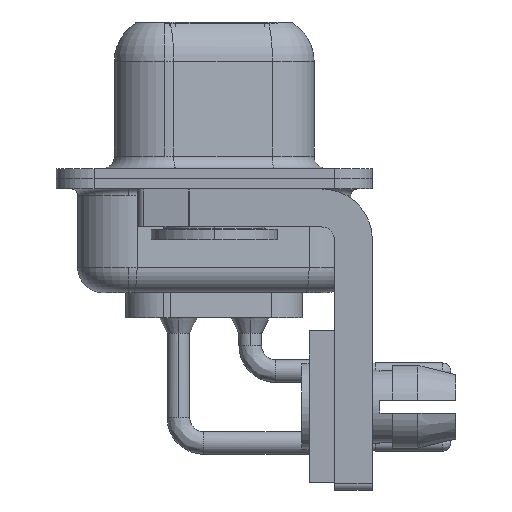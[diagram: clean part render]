
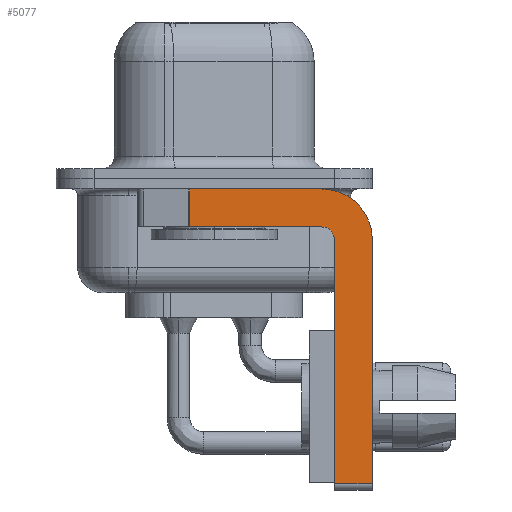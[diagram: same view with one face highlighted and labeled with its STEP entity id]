
A CAD part, left-side view. The second image highlights one B-rep face of the part: STEP entity #5077.
In plain terms, the highlighted planar face has unit normal (-1, 0, 0).
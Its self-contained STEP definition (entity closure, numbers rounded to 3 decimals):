
#413 = DIRECTION ( 'NONE',  ( 0., -1., 0. ) ) ;
#438 = EDGE_CURVE ( 'NONE', #1953, #17563, #21297, .T. ) ;
#476 = AXIS2_PLACEMENT_3D ( 'NONE', #9005, #9037, #8812 ) ;
#985 = CIRCLE ( 'NONE', #476, 2. ) ;
#1953 = VERTEX_POINT ( 'NONE', #21145 ) ;
#1963 = EDGE_CURVE ( 'NONE', #9239, #7522, #6109, .T. ) ;
#2119 = AXIS2_PLACEMENT_3D ( 'NONE', #20355, #21916, #20970 ) ;
#2175 = EDGE_CURVE ( 'NONE', #17563, #11756, #985, .T. ) ;
#2285 = LINE ( 'NONE', #16053, #13680 ) ;
#2563 = DIRECTION ( 'NONE',  ( 0., 0., -1. ) ) ;
#2625 = CARTESIAN_POINT ( 'NONE',  ( -2.9, -4.25, -0.4 ) ) ;
#2735 = VERTEX_POINT ( 'NONE', #4175 ) ;
#3750 = VECTOR ( 'NONE', #413, 1000. ) ;
#3784 = ORIENTED_EDGE ( 'NONE', *, *, #438, .F. ) ;
#3963 = EDGE_CURVE ( 'NONE', #6126, #12973, #21067, .T. ) ;
#4175 = CARTESIAN_POINT ( 'NONE',  ( -2.9, 0.978, -1.9 ) ) ;
#5077 = ADVANCED_FACE ( 'NONE', ( #16055 ), #5805, .F. ) ;
#5805 = PLANE ( 'NONE',  #9897 ) ;
#5872 = CARTESIAN_POINT ( 'NONE',  ( -2.9, -4.25, -2.4 ) ) ;
#6109 = CIRCLE ( 'NONE', #2119, 0.5 ) ;
#6126 = VERTEX_POINT ( 'NONE', #13852 ) ;
#6185 = DIRECTION ( 'NONE',  ( 0., 0., -1. ) ) ;
#6246 = DIRECTION ( 'NONE',  ( 1., 0., 0. ) ) ;
#6456 = ORIENTED_EDGE ( 'NONE', *, *, #13856, .F. ) ;
#6902 = CARTESIAN_POINT ( 'NONE',  ( -2.9, 3., -0.4 ) ) ;
#7522 = VERTEX_POINT ( 'NONE', #16894 ) ;
#7838 = EDGE_CURVE ( 'NONE', #11756, #12973, #2285, .T. ) ;
#8098 = ORIENTED_EDGE ( 'NONE', *, *, #3963, .T. ) ;
#8130 = LINE ( 'NONE', #17653, #8649 ) ;
#8649 = VECTOR ( 'NONE', #9329, 1000. ) ;
#8812 = DIRECTION ( 'NONE',  ( 0., 0., -1. ) ) ;
#9005 = CARTESIAN_POINT ( 'NONE',  ( -2.9, -4.25, -2.4 ) ) ;
#9037 = DIRECTION ( 'NONE',  ( 1., 0., 0. ) ) ;
#9053 = EDGE_CURVE ( 'NONE', #1953, #2735, #8130, .T. ) ;
#9165 = DIRECTION ( 'NONE',  ( 0., 1., 0. ) ) ;
#9239 = VERTEX_POINT ( 'NONE', #13207 ) ;
#9329 = DIRECTION ( 'NONE',  ( 0., 0., -1. ) ) ;
#9823 = VECTOR ( 'NONE', #9165, 1000. ) ;
#9897 = AXIS2_PLACEMENT_3D ( 'NONE', #5872, #6246, #6185 ) ;
#11756 = VERTEX_POINT ( 'NONE', #12851 ) ;
#12767 = CARTESIAN_POINT ( 'NONE',  ( -2.9, -4.25, -12.05 ) ) ;
#12851 = CARTESIAN_POINT ( 'NONE',  ( -2.9, -6.25, -2.4 ) ) ;
#12973 = VERTEX_POINT ( 'NONE', #18842 ) ;
#13011 = DIRECTION ( 'NONE',  ( 0., -1., 0. ) ) ;
#13207 = CARTESIAN_POINT ( 'NONE',  ( -2.9, -4.75, -2.4 ) ) ;
#13386 = ORIENTED_EDGE ( 'NONE', *, *, #2175, .F. ) ;
#13680 = VECTOR ( 'NONE', #2563, 1000. ) ;
#13852 = CARTESIAN_POINT ( 'NONE',  ( -2.9, -4.75, -12.05 ) ) ;
#13856 = EDGE_CURVE ( 'NONE', #7522, #2735, #18695, .T. ) ;
#14243 = VECTOR ( 'NONE', #21085, 1000. ) ;
#14579 = ORIENTED_EDGE ( 'NONE', *, *, #1963, .F. ) ;
#15173 = ORIENTED_EDGE ( 'NONE', *, *, #18150, .F. ) ;
#16053 = CARTESIAN_POINT ( 'NONE',  ( -2.9, -6.25, -2.4 ) ) ;
#16055 = FACE_OUTER_BOUND ( 'NONE', #18498, .T. ) ;
#16894 = CARTESIAN_POINT ( 'NONE',  ( -2.9, -4.25, -1.9 ) ) ;
#17563 = VERTEX_POINT ( 'NONE', #2625 ) ;
#17653 = CARTESIAN_POINT ( 'NONE',  ( -2.9, 0.978, -1.9 ) ) ;
#18150 = EDGE_CURVE ( 'NONE', #6126, #9239, #18658, .T. ) ;
#18202 = ORIENTED_EDGE ( 'NONE', *, *, #9053, .T. ) ;
#18498 = EDGE_LOOP ( 'NONE', ( #3784, #18202, #6456, #14579, #15173, #8098, #21964, #13386 ) ) ;
#18658 = LINE ( 'NONE', #21017, #14243 ) ;
#18695 = LINE ( 'NONE', #20850, #9823 ) ;
#18842 = CARTESIAN_POINT ( 'NONE',  ( -2.9, -6.25, -12.05 ) ) ;
#20355 = CARTESIAN_POINT ( 'NONE',  ( -2.9, -4.25, -2.4 ) ) ;
#20850 = CARTESIAN_POINT ( 'NONE',  ( -2.9, -4.25, -1.9 ) ) ;
#20970 = DIRECTION ( 'NONE',  ( 0., 0., 1. ) ) ;
#21017 = CARTESIAN_POINT ( 'NONE',  ( -2.9, -4.75, -12.3 ) ) ;
#21067 = LINE ( 'NONE', #12767, #3750 ) ;
#21085 = DIRECTION ( 'NONE',  ( 0., 0., 1. ) ) ;
#21145 = CARTESIAN_POINT ( 'NONE',  ( -2.9, 0.978, -0.4 ) ) ;
#21297 = LINE ( 'NONE', #6902, #21856 ) ;
#21856 = VECTOR ( 'NONE', #13011, 1000. ) ;
#21916 = DIRECTION ( 'NONE',  ( -1., 0., 0. ) ) ;
#21964 = ORIENTED_EDGE ( 'NONE', *, *, #7838, .F. ) ;
